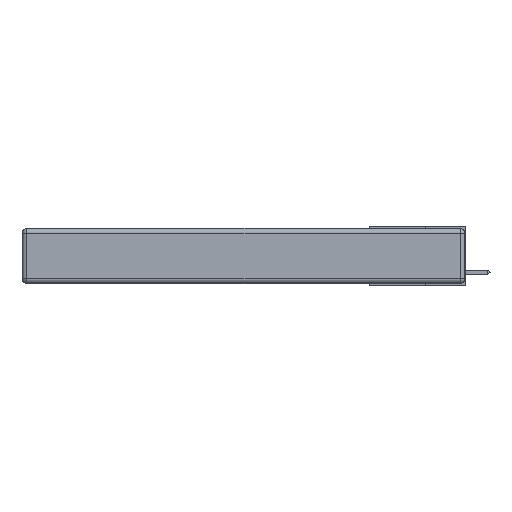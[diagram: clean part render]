
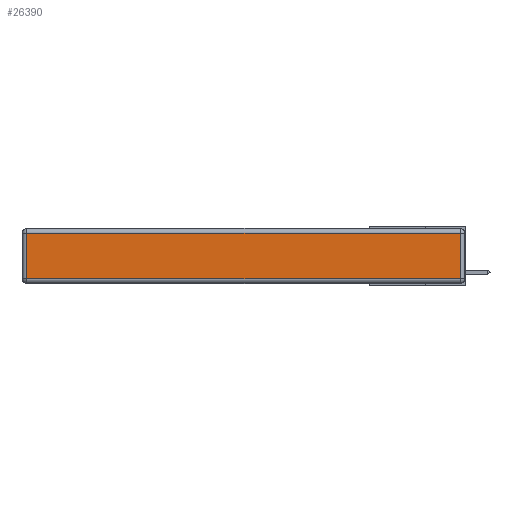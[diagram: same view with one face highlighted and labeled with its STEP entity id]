
A CAD part, left-side view. The second image highlights one B-rep face of the part: STEP entity #26390.
In plain terms, the highlighted planar face has unit normal (-1, 0, 0).
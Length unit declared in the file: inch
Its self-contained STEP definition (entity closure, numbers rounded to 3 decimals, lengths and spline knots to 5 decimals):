
#513 = EDGE_CURVE ( 'NONE', #11185, #23077, #22509, .T. ) ;
#1528 = CARTESIAN_POINT ( 'NONE',  ( 0., 0.03, -0.03 ) ) ;
#2519 = DIRECTION ( 'NONE',  ( 0., 0., -1. ) ) ;
#4019 = DIRECTION ( 'NONE',  ( 0., 0., 1. ) ) ;
#4293 = CARTESIAN_POINT ( 'NONE',  ( 0., 2.72, -0.313 ) ) ;
#4561 = EDGE_LOOP ( 'NONE', ( #20170, #29106, #4657, #6424 ) ) ;
#4657 = ORIENTED_EDGE ( 'NONE', *, *, #513, .T. ) ;
#4837 = CARTESIAN_POINT ( 'NONE',  ( 0., 0.03, -0.313 ) ) ;
#5058 = CARTESIAN_POINT ( 'NONE',  ( 0., 2.75, -0.03 ) ) ;
#5241 = EDGE_CURVE ( 'NONE', #28185, #10372, #28917, .T. ) ;
#6424 = ORIENTED_EDGE ( 'NONE', *, *, #20851, .T. ) ;
#7069 = DIRECTION ( 'NONE',  ( 0., 1., 0. ) ) ;
#8400 = CARTESIAN_POINT ( 'NONE',  ( 0., 2.72, -0.03 ) ) ;
#8576 = LINE ( 'NONE', #28547, #28999 ) ;
#8792 = VECTOR ( 'NONE', #2519, 39.37008 ) ;
#9710 = AXIS2_PLACEMENT_3D ( 'NONE', #12458, #26172, #4019 ) ;
#10152 = PLANE ( 'NONE',  #9710 ) ;
#10372 = VERTEX_POINT ( 'NONE', #4837 ) ;
#11185 = VERTEX_POINT ( 'NONE', #1528 ) ;
#12458 = CARTESIAN_POINT ( 'NONE',  ( 0., 0., -0.343 ) ) ;
#12727 = DIRECTION ( 'NONE',  ( 0., 0., 1. ) ) ;
#16750 = VECTOR ( 'NONE', #28426, 39.37008 ) ;
#17430 = CARTESIAN_POINT ( 'NONE',  ( 0., 0., -0.313 ) ) ;
#17930 = FACE_OUTER_BOUND ( 'NONE', #4561, .T. ) ;
#20170 = ORIENTED_EDGE ( 'NONE', *, *, #5241, .T. ) ;
#20236 = LINE ( 'NONE', #20777, #8792 ) ;
#20777 = CARTESIAN_POINT ( 'NONE',  ( 0., 2.72, -0.343 ) ) ;
#20851 = EDGE_CURVE ( 'NONE', #23077, #28185, #20236, .T. ) ;
#22509 = LINE ( 'NONE', #5058, #25387 ) ;
#23077 = VERTEX_POINT ( 'NONE', #8400 ) ;
#25387 = VECTOR ( 'NONE', #7069, 39.37008 ) ;
#26172 = DIRECTION ( 'NONE',  ( -1., 0., 0. ) ) ;
#26390 = ADVANCED_FACE ( 'NONE', ( #17930 ), #10152, .T. ) ;
#26894 = EDGE_CURVE ( 'NONE', #10372, #11185, #8576, .T. ) ;
#28185 = VERTEX_POINT ( 'NONE', #4293 ) ;
#28426 = DIRECTION ( 'NONE',  ( 0., -1., 0. ) ) ;
#28547 = CARTESIAN_POINT ( 'NONE',  ( 0., 0.03, -0.343 ) ) ;
#28917 = LINE ( 'NONE', #17430, #16750 ) ;
#28999 = VECTOR ( 'NONE', #12727, 39.37008 ) ;
#29106 = ORIENTED_EDGE ( 'NONE', *, *, #26894, .T. ) ;
